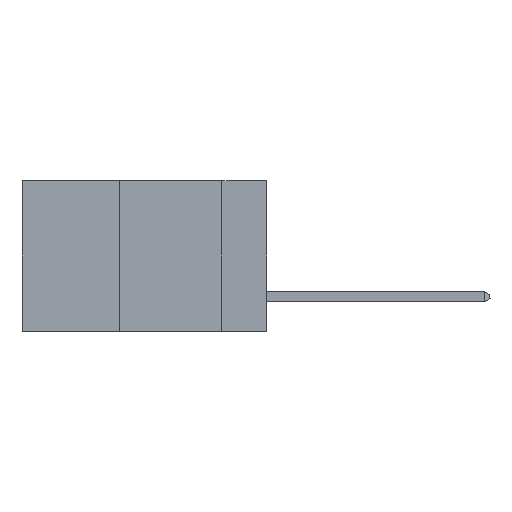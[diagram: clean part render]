
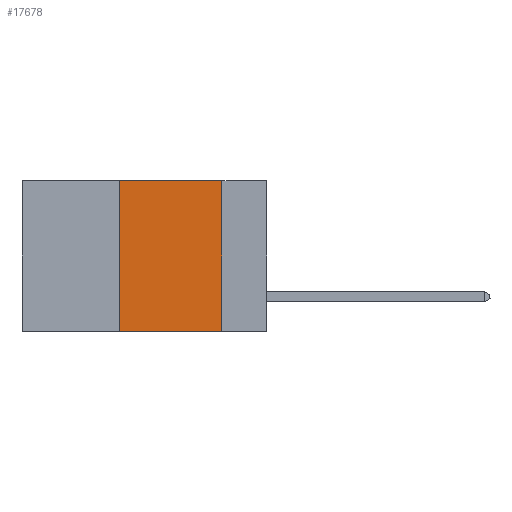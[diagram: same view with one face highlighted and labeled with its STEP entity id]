
A CAD part, left-side view. The second image highlights one B-rep face of the part: STEP entity #17678.
In plain terms, the highlighted planar face has unit normal (-1, 0, 0).
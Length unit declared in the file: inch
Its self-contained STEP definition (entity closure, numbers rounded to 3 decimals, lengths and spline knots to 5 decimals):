
#308 = CARTESIAN_POINT ( 'NONE',  ( 0., 0.11, 0. ) ) ;
#502 = CARTESIAN_POINT ( 'NONE',  ( 0., 0.11, 0. ) ) ;
#1135 = CARTESIAN_POINT ( 'NONE',  ( 0., 0.6, 0. ) ) ;
#1188 = LINE ( 'NONE', #16016, #1880 ) ;
#1686 = CARTESIAN_POINT ( 'NONE',  ( 0., 0.36, 0. ) ) ;
#1807 = DIRECTION ( 'NONE',  ( 0., 0., -1. ) ) ;
#1880 = VECTOR ( 'NONE', #7337, 39.37008 ) ;
#2763 = VECTOR ( 'NONE', #18603, 39.37008 ) ;
#3164 = EDGE_CURVE ( 'NONE', #8270, #3478, #17061, .T. ) ;
#3478 = VERTEX_POINT ( 'NONE', #502 ) ;
#3977 = AXIS2_PLACEMENT_3D ( 'NONE', #11746, #5817, #8701 ) ;
#4584 = EDGE_CURVE ( 'NONE', #3478, #10883, #15907, .T. ) ;
#4787 = VERTEX_POINT ( 'NONE', #9870 ) ;
#5444 = VECTOR ( 'NONE', #14459, 39.37008 ) ;
#5817 = DIRECTION ( 'NONE',  ( 1., 0., 0. ) ) ;
#5996 = CARTESIAN_POINT ( 'NONE',  ( 0., 0.36, 0. ) ) ;
#6380 = CARTESIAN_POINT ( 'NONE',  ( 0., 0.11, -0.37 ) ) ;
#6604 = ORIENTED_EDGE ( 'NONE', *, *, #3164, .F. ) ;
#6830 = LINE ( 'NONE', #1686, #5444 ) ;
#7337 = DIRECTION ( 'NONE',  ( 0., -1., 0. ) ) ;
#7491 = PLANE ( 'NONE',  #3977 ) ;
#8270 = VERTEX_POINT ( 'NONE', #5996 ) ;
#8701 = DIRECTION ( 'NONE',  ( 0., 0., -1. ) ) ;
#8742 = EDGE_CURVE ( 'NONE', #4787, #10883, #1188, .T. ) ;
#9557 = ORIENTED_EDGE ( 'NONE', *, *, #10101, .F. ) ;
#9870 = CARTESIAN_POINT ( 'NONE',  ( 0., 0.36, -0.37 ) ) ;
#10101 = EDGE_CURVE ( 'NONE', #4787, #8270, #6830, .T. ) ;
#10477 = ORIENTED_EDGE ( 'NONE', *, *, #4584, .F. ) ;
#10883 = VERTEX_POINT ( 'NONE', #6380 ) ;
#11746 = CARTESIAN_POINT ( 'NONE',  ( 0., 0.6, 0. ) ) ;
#12112 = FACE_OUTER_BOUND ( 'NONE', #13758, .T. ) ;
#13758 = EDGE_LOOP ( 'NONE', ( #10477, #6604, #9557, #15661 ) ) ;
#14459 = DIRECTION ( 'NONE',  ( 0., 0., 1. ) ) ;
#15661 = ORIENTED_EDGE ( 'NONE', *, *, #8742, .T. ) ;
#15907 = LINE ( 'NONE', #308, #16812 ) ;
#16016 = CARTESIAN_POINT ( 'NONE',  ( 0., 0.6, -0.37 ) ) ;
#16812 = VECTOR ( 'NONE', #1807, 39.37008 ) ;
#17061 = LINE ( 'NONE', #1135, #2763 ) ;
#17678 = ADVANCED_FACE ( 'NONE', ( #12112 ), #7491, .F. ) ;
#18603 = DIRECTION ( 'NONE',  ( 0., -1., 0. ) ) ;
